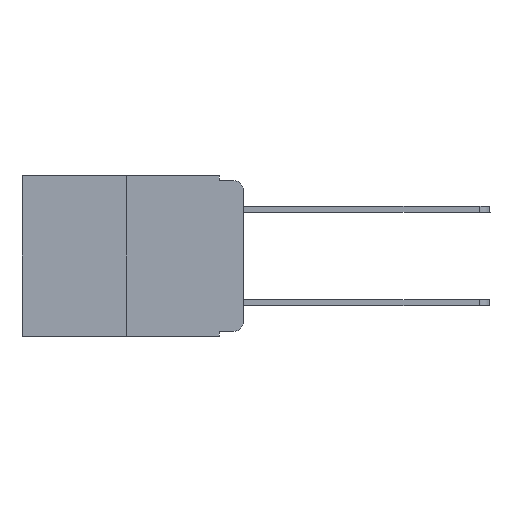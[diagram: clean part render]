
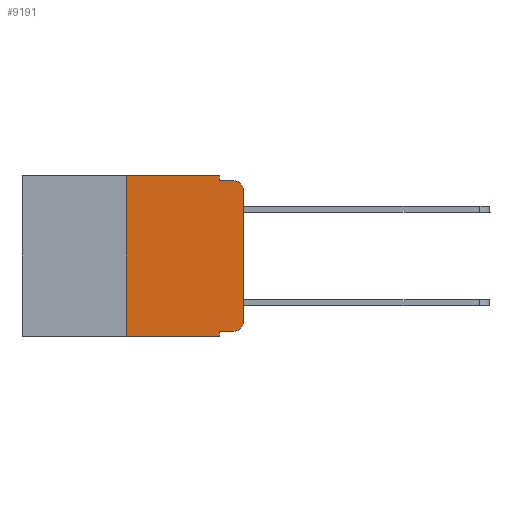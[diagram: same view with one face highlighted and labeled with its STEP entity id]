
A CAD part, left-side view. The second image highlights one B-rep face of the part: STEP entity #9191.
In plain terms, the highlighted planar face has unit normal (-1, 0, 0).
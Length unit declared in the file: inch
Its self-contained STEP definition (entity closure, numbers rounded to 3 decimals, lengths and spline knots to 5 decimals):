
#107 = EDGE_CURVE ( 'NONE', #22002, #11418, #418, .T. ) ;
#359 = CARTESIAN_POINT ( 'NONE',  ( 0., 0.473, 0. ) ) ;
#418 = LINE ( 'NONE', #5785, #4611 ) ;
#679 = DIRECTION ( 'NONE',  ( 0., -1., 0. ) ) ;
#756 = CARTESIAN_POINT ( 'NONE',  ( 0., 0.051, -0.01 ) ) ;
#1082 = ORIENTED_EDGE ( 'NONE', *, *, #22540, .F. ) ;
#1360 = CARTESIAN_POINT ( 'NONE',  ( 0., 0.02, -0.333 ) ) ;
#1806 = EDGE_CURVE ( 'NONE', #14135, #2515, #17419, .T. ) ;
#1911 = CIRCLE ( 'NONE', #22289, 0.02 ) ;
#1927 = CARTESIAN_POINT ( 'NONE',  ( 0., 0.02, -0.313 ) ) ;
#2394 = CARTESIAN_POINT ( 'NONE',  ( 0., 0.051, 0. ) ) ;
#2426 = AXIS2_PLACEMENT_3D ( 'NONE', #10211, #19051, #13612 ) ;
#2515 = VERTEX_POINT ( 'NONE', #5182 ) ;
#3330 = EDGE_CURVE ( 'NONE', #11418, #10649, #1911, .T. ) ;
#3720 = DIRECTION ( 'NONE',  ( 0., -1., 0. ) ) ;
#3813 = DIRECTION ( 'NONE',  ( 0., 0., -1. ) ) ;
#3956 = LINE ( 'NONE', #2394, #13525 ) ;
#4450 = EDGE_CURVE ( 'NONE', #17015, #14495, #12855, .T. ) ;
#4611 = VECTOR ( 'NONE', #5863, 39.37008 ) ;
#4725 = PLANE ( 'NONE',  #2426 ) ;
#4897 = CARTESIAN_POINT ( 'NONE',  ( 0., 0.051, 0. ) ) ;
#4933 = ORIENTED_EDGE ( 'NONE', *, *, #16177, .F. ) ;
#5182 = CARTESIAN_POINT ( 'NONE',  ( 0., 0.051, -0.01 ) ) ;
#5333 = ORIENTED_EDGE ( 'NONE', *, *, #4450, .T. ) ;
#5493 = VECTOR ( 'NONE', #17676, 39.37008 ) ;
#5608 = CARTESIAN_POINT ( 'NONE',  ( 0., 0., 0. ) ) ;
#5785 = CARTESIAN_POINT ( 'NONE',  ( 0., 0.051, -0.333 ) ) ;
#5863 = DIRECTION ( 'NONE',  ( 0., -1., 0. ) ) ;
#7266 = DIRECTION ( 'NONE',  ( -1., 0., 0. ) ) ;
#7308 = VECTOR ( 'NONE', #10787, 39.37008 ) ;
#7631 = ORIENTED_EDGE ( 'NONE', *, *, #9432, .T. ) ;
#7644 = ORIENTED_EDGE ( 'NONE', *, *, #107, .T. ) ;
#7819 = CARTESIAN_POINT ( 'NONE',  ( 0., 0., -0.313 ) ) ;
#8050 = AXIS2_PLACEMENT_3D ( 'NONE', #10173, #13578, #11936 ) ;
#8782 = LINE ( 'NONE', #5608, #10186 ) ;
#9137 = LINE ( 'NONE', #21346, #5493 ) ;
#9191 = ADVANCED_FACE ( 'NONE', ( #22817 ), #4725, .F. ) ;
#9432 = EDGE_CURVE ( 'NONE', #10649, #17015, #8782, .T. ) ;
#10173 = CARTESIAN_POINT ( 'NONE',  ( 0., 0.02, -0.03 ) ) ;
#10186 = VECTOR ( 'NONE', #16359, 39.37008 ) ;
#10211 = CARTESIAN_POINT ( 'NONE',  ( 0., 0.473, 0. ) ) ;
#10649 = VERTEX_POINT ( 'NONE', #7819 ) ;
#10721 = VERTEX_POINT ( 'NONE', #22649 ) ;
#10787 = DIRECTION ( 'NONE',  ( 0., -1., 0. ) ) ;
#11095 = VERTEX_POINT ( 'NONE', #11909 ) ;
#11418 = VERTEX_POINT ( 'NONE', #1360 ) ;
#11740 = EDGE_CURVE ( 'NONE', #10721, #14135, #19465, .T. ) ;
#11909 = CARTESIAN_POINT ( 'NONE',  ( 0., 0.051, -0.343 ) ) ;
#11936 = DIRECTION ( 'NONE',  ( 0., 0., -1. ) ) ;
#11977 = ORIENTED_EDGE ( 'NONE', *, *, #1806, .F. ) ;
#12855 = CIRCLE ( 'NONE', #8050, 0.02 ) ;
#13525 = VECTOR ( 'NONE', #15103, 39.37008 ) ;
#13578 = DIRECTION ( 'NONE',  ( -1., 0., 0. ) ) ;
#13612 = DIRECTION ( 'NONE',  ( 0., 0., -1. ) ) ;
#13629 = DIRECTION ( 'NONE',  ( 0., 0., -1. ) ) ;
#13659 = CARTESIAN_POINT ( 'NONE',  ( 0., 0.051, -0.333 ) ) ;
#13953 = EDGE_CURVE ( 'NONE', #2515, #14495, #22152, .T. ) ;
#14135 = VERTEX_POINT ( 'NONE', #4897 ) ;
#14495 = VERTEX_POINT ( 'NONE', #14551 ) ;
#14551 = CARTESIAN_POINT ( 'NONE',  ( 0., 0.02, -0.01 ) ) ;
#14574 = ORIENTED_EDGE ( 'NONE', *, *, #11740, .F. ) ;
#14637 = VECTOR ( 'NONE', #679, 39.37008 ) ;
#15103 = DIRECTION ( 'NONE',  ( 0., 0., -1. ) ) ;
#16177 = EDGE_CURVE ( 'NONE', #19816, #10721, #9137, .T. ) ;
#16359 = DIRECTION ( 'NONE',  ( 0., 0., 1. ) ) ;
#17015 = VERTEX_POINT ( 'NONE', #18116 ) ;
#17251 = EDGE_LOOP ( 'NONE', ( #7631, #5333, #21063, #11977, #14574, #4933, #20336, #1082, #7644, #17924 ) ) ;
#17419 = LINE ( 'NONE', #22544, #21884 ) ;
#17676 = DIRECTION ( 'NONE',  ( 0., 0., 1. ) ) ;
#17924 = ORIENTED_EDGE ( 'NONE', *, *, #3330, .T. ) ;
#18116 = CARTESIAN_POINT ( 'NONE',  ( 0., 0., -0.03 ) ) ;
#18154 = CARTESIAN_POINT ( 'NONE',  ( 0., 0.25, -0.343 ) ) ;
#18616 = VECTOR ( 'NONE', #3720, 39.37008 ) ;
#19051 = DIRECTION ( 'NONE',  ( 1., 0., 0. ) ) ;
#19465 = LINE ( 'NONE', #359, #18616 ) ;
#19816 = VERTEX_POINT ( 'NONE', #18154 ) ;
#20336 = ORIENTED_EDGE ( 'NONE', *, *, #22993, .T. ) ;
#21063 = ORIENTED_EDGE ( 'NONE', *, *, #13953, .F. ) ;
#21346 = CARTESIAN_POINT ( 'NONE',  ( 0., 0.25, 0. ) ) ;
#21649 = CARTESIAN_POINT ( 'NONE',  ( 0., 0.473, -0.343 ) ) ;
#21869 = LINE ( 'NONE', #21649, #7308 ) ;
#21884 = VECTOR ( 'NONE', #13629, 39.37008 ) ;
#22002 = VERTEX_POINT ( 'NONE', #13659 ) ;
#22152 = LINE ( 'NONE', #756, #14637 ) ;
#22289 = AXIS2_PLACEMENT_3D ( 'NONE', #1927, #7266, #3813 ) ;
#22540 = EDGE_CURVE ( 'NONE', #22002, #11095, #3956, .T. ) ;
#22544 = CARTESIAN_POINT ( 'NONE',  ( 0., 0.051, 0. ) ) ;
#22649 = CARTESIAN_POINT ( 'NONE',  ( 0., 0.25, 0. ) ) ;
#22817 = FACE_OUTER_BOUND ( 'NONE', #17251, .T. ) ;
#22993 = EDGE_CURVE ( 'NONE', #19816, #11095, #21869, .T. ) ;
